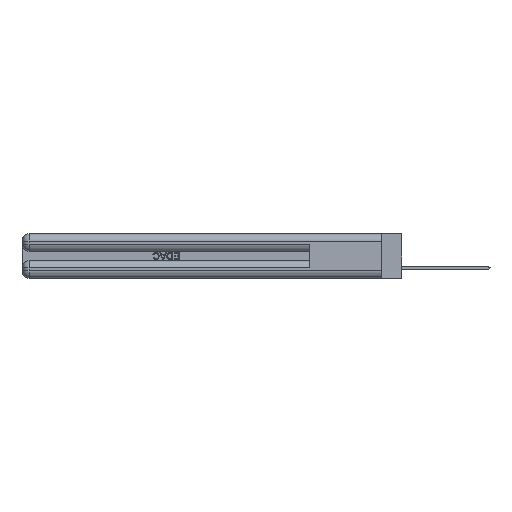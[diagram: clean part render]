
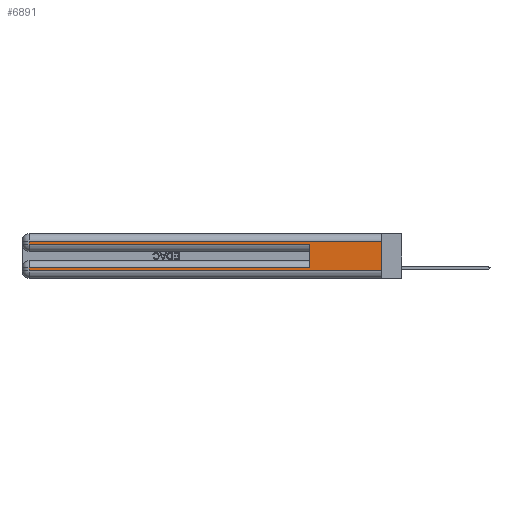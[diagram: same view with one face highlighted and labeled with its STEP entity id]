
A CAD part, left-side view. The second image highlights one B-rep face of the part: STEP entity #6891.
In plain terms, the highlighted planar face has unit normal (-1, 0, 0).
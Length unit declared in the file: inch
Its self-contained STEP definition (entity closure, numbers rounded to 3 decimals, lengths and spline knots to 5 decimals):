
#198 = CARTESIAN_POINT ( 'NONE',  ( 0., 0.6, 0.285 ) ) ;
#837 = CARTESIAN_POINT ( 'NONE',  ( 0., 2.94, 0.085 ) ) ;
#919 = EDGE_CURVE ( 'NONE', #23200, #43053, #33432, .T. ) ;
#1436 = VECTOR ( 'NONE', #33790, 39.37008 ) ;
#1663 = VERTEX_POINT ( 'NONE', #41167 ) ;
#1713 = VERTEX_POINT ( 'NONE', #198 ) ;
#2580 = VERTEX_POINT ( 'NONE', #29282 ) ;
#3978 = DIRECTION ( 'NONE',  ( 0., -1., 0. ) ) ;
#4627 = VECTOR ( 'NONE', #3978, 39.37008 ) ;
#5662 = CARTESIAN_POINT ( 'NONE',  ( 0., 0., 0.085 ) ) ;
#5800 = VECTOR ( 'NONE', #19265, 39.37008 ) ;
#6431 = ORIENTED_EDGE ( 'NONE', *, *, #36323, .T. ) ;
#6656 = CARTESIAN_POINT ( 'NONE',  ( 0., 0., 0.06 ) ) ;
#6891 = ADVANCED_FACE ( 'NONE', ( #14399 ), #43158, .F. ) ;
#6976 = DIRECTION ( 'NONE',  ( 1., 0., 0. ) ) ;
#7274 = VECTOR ( 'NONE', #23518, 39.37008 ) ;
#7670 = ORIENTED_EDGE ( 'NONE', *, *, #31572, .T. ) ;
#7817 = LINE ( 'NONE', #23375, #7274 ) ;
#9982 = DIRECTION ( 'NONE',  ( 0., 1., 0. ) ) ;
#11968 = EDGE_CURVE ( 'NONE', #42671, #2580, #12283, .T. ) ;
#12145 = CARTESIAN_POINT ( 'NONE',  ( 0., 0., 0.31 ) ) ;
#12283 = LINE ( 'NONE', #20250, #20289 ) ;
#12554 = EDGE_CURVE ( 'NONE', #42671, #43053, #24021, .T. ) ;
#12906 = ORIENTED_EDGE ( 'NONE', *, *, #36783, .F. ) ;
#13290 = ORIENTED_EDGE ( 'NONE', *, *, #919, .T. ) ;
#14399 = FACE_OUTER_BOUND ( 'NONE', #17315, .T. ) ;
#14752 = LINE ( 'NONE', #18019, #22793 ) ;
#15879 = VERTEX_POINT ( 'NONE', #837 ) ;
#16078 = DIRECTION ( 'NONE',  ( 0., 1., 0. ) ) ;
#16211 = CARTESIAN_POINT ( 'NONE',  ( 0., 0., 0.37 ) ) ;
#17315 = EDGE_LOOP ( 'NONE', ( #38851, #31522, #39667, #6431, #12906, #7670, #36756, #13290 ) ) ;
#17930 = CARTESIAN_POINT ( 'NONE',  ( 0., 2.94, 0.37 ) ) ;
#18019 = CARTESIAN_POINT ( 'NONE',  ( 0., 2.94, 0.37 ) ) ;
#18159 = DIRECTION ( 'NONE',  ( 0., 0., -1. ) ) ;
#19265 = DIRECTION ( 'NONE',  ( 0., 0., -1. ) ) ;
#19950 = LINE ( 'NONE', #5662, #43940 ) ;
#20250 = CARTESIAN_POINT ( 'NONE',  ( 0., 0., 0.31 ) ) ;
#20289 = VECTOR ( 'NONE', #9982, 39.37008 ) ;
#20380 = DIRECTION ( 'NONE',  ( 0., 0., -1. ) ) ;
#22793 = VECTOR ( 'NONE', #18159, 39.37008 ) ;
#22836 = LINE ( 'NONE', #17930, #5800 ) ;
#23200 = VERTEX_POINT ( 'NONE', #42613 ) ;
#23337 = LINE ( 'NONE', #24418, #4627 ) ;
#23375 = CARTESIAN_POINT ( 'NONE',  ( 0., 0.6, 0.145 ) ) ;
#23518 = DIRECTION ( 'NONE',  ( 0., 0., 1. ) ) ;
#24021 = LINE ( 'NONE', #35569, #26682 ) ;
#24418 = CARTESIAN_POINT ( 'NONE',  ( 0., 0., 0.285 ) ) ;
#26682 = VECTOR ( 'NONE', #42411, 39.37008 ) ;
#29282 = CARTESIAN_POINT ( 'NONE',  ( 0., 2.94, 0.31 ) ) ;
#31479 = VERTEX_POINT ( 'NONE', #38776 ) ;
#31522 = ORIENTED_EDGE ( 'NONE', *, *, #11968, .T. ) ;
#31572 = EDGE_CURVE ( 'NONE', #31479, #15879, #19950, .T. ) ;
#33432 = LINE ( 'NONE', #6656, #1436 ) ;
#33790 = DIRECTION ( 'NONE',  ( 0., -1., 0. ) ) ;
#35569 = CARTESIAN_POINT ( 'NONE',  ( 0., 0., 0.37 ) ) ;
#35773 = EDGE_CURVE ( 'NONE', #2580, #1663, #14752, .T. ) ;
#36323 = EDGE_CURVE ( 'NONE', #1663, #1713, #23337, .T. ) ;
#36756 = ORIENTED_EDGE ( 'NONE', *, *, #42600, .T. ) ;
#36783 = EDGE_CURVE ( 'NONE', #31479, #1713, #7817, .T. ) ;
#38561 = AXIS2_PLACEMENT_3D ( 'NONE', #16211, #6976, #20380 ) ;
#38776 = CARTESIAN_POINT ( 'NONE',  ( 0., 0.6, 0.085 ) ) ;
#38851 = ORIENTED_EDGE ( 'NONE', *, *, #12554, .F. ) ;
#39667 = ORIENTED_EDGE ( 'NONE', *, *, #35773, .T. ) ;
#41167 = CARTESIAN_POINT ( 'NONE',  ( 0., 2.94, 0.285 ) ) ;
#41416 = CARTESIAN_POINT ( 'NONE',  ( 0., 0., 0.06 ) ) ;
#42411 = DIRECTION ( 'NONE',  ( 0., 0., -1. ) ) ;
#42600 = EDGE_CURVE ( 'NONE', #15879, #23200, #22836, .T. ) ;
#42613 = CARTESIAN_POINT ( 'NONE',  ( 0., 2.94, 0.06 ) ) ;
#42671 = VERTEX_POINT ( 'NONE', #12145 ) ;
#43053 = VERTEX_POINT ( 'NONE', #41416 ) ;
#43158 = PLANE ( 'NONE',  #38561 ) ;
#43940 = VECTOR ( 'NONE', #16078, 39.37008 ) ;
